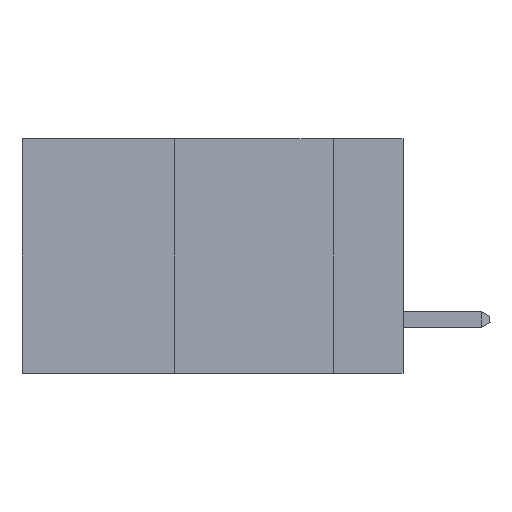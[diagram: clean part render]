
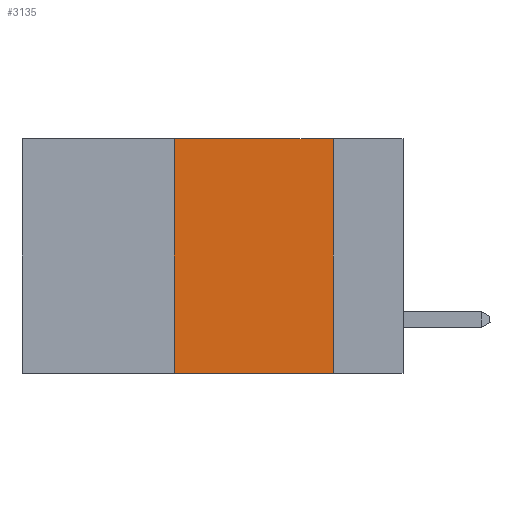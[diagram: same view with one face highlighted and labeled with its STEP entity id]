
A CAD part, left-side view. The second image highlights one B-rep face of the part: STEP entity #3135.
In plain terms, the highlighted planar face has unit normal (-1, 0, 0).
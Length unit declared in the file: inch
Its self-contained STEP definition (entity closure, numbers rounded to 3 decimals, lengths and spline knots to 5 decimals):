
#209 = VERTEX_POINT ( 'NONE', #3445 ) ;
#463 = CARTESIAN_POINT ( 'NONE',  ( 0., 0.11, 0. ) ) ;
#902 = CARTESIAN_POINT ( 'NONE',  ( 0., 0.6, 0. ) ) ;
#1029 = EDGE_CURVE ( 'NONE', #12218, #3505, #1140, .T. ) ;
#1140 = LINE ( 'NONE', #902, #3701 ) ;
#1159 = EDGE_CURVE ( 'NONE', #7210, #209, #2060, .T. ) ;
#1378 = ORIENTED_EDGE ( 'NONE', *, *, #1628, .F. ) ;
#1628 = EDGE_CURVE ( 'NONE', #7210, #12218, #4470, .T. ) ;
#1922 = CARTESIAN_POINT ( 'NONE',  ( 0., 0.6, -0.37 ) ) ;
#1966 = DIRECTION ( 'NONE',  ( 0., -1., 0. ) ) ;
#2060 = LINE ( 'NONE', #1922, #11329 ) ;
#2208 = LINE ( 'NONE', #10296, #12258 ) ;
#2541 = DIRECTION ( 'NONE',  ( 1., 0., 0. ) ) ;
#3135 = ADVANCED_FACE ( 'NONE', ( #6265 ), #9269, .F. ) ;
#3384 = VECTOR ( 'NONE', #4978, 39.37008 ) ;
#3445 = CARTESIAN_POINT ( 'NONE',  ( 0., 0.11, -0.37 ) ) ;
#3505 = VERTEX_POINT ( 'NONE', #463 ) ;
#3558 = AXIS2_PLACEMENT_3D ( 'NONE', #5613, #2541, #4646 ) ;
#3611 = ORIENTED_EDGE ( 'NONE', *, *, #1029, .F. ) ;
#3701 = VECTOR ( 'NONE', #11615, 39.37008 ) ;
#4470 = LINE ( 'NONE', #12550, #3384 ) ;
#4646 = DIRECTION ( 'NONE',  ( 0., 0., -1. ) ) ;
#4935 = ORIENTED_EDGE ( 'NONE', *, *, #1159, .T. ) ;
#4978 = DIRECTION ( 'NONE',  ( 0., 0., 1. ) ) ;
#5613 = CARTESIAN_POINT ( 'NONE',  ( 0., 0.6, 0. ) ) ;
#6265 = FACE_OUTER_BOUND ( 'NONE', #7873, .T. ) ;
#6267 = ORIENTED_EDGE ( 'NONE', *, *, #9284, .F. ) ;
#7210 = VERTEX_POINT ( 'NONE', #12366 ) ;
#7873 = EDGE_LOOP ( 'NONE', ( #6267, #3611, #1378, #4935 ) ) ;
#8413 = DIRECTION ( 'NONE',  ( 0., 0., -1. ) ) ;
#9269 = PLANE ( 'NONE',  #3558 ) ;
#9284 = EDGE_CURVE ( 'NONE', #3505, #209, #2208, .T. ) ;
#9403 = CARTESIAN_POINT ( 'NONE',  ( 0., 0.36, 0. ) ) ;
#10296 = CARTESIAN_POINT ( 'NONE',  ( 0., 0.11, 0. ) ) ;
#11329 = VECTOR ( 'NONE', #1966, 39.37008 ) ;
#11615 = DIRECTION ( 'NONE',  ( 0., -1., 0. ) ) ;
#12218 = VERTEX_POINT ( 'NONE', #9403 ) ;
#12258 = VECTOR ( 'NONE', #8413, 39.37008 ) ;
#12366 = CARTESIAN_POINT ( 'NONE',  ( 0., 0.36, -0.37 ) ) ;
#12550 = CARTESIAN_POINT ( 'NONE',  ( 0., 0.36, 0. ) ) ;
